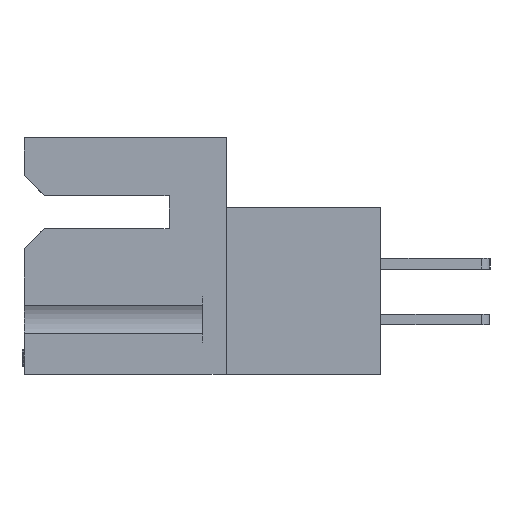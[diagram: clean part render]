
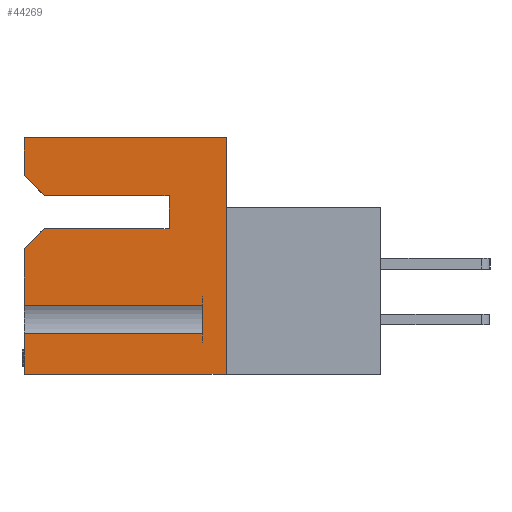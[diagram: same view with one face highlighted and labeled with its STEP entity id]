
A CAD part, left-side view. The second image highlights one B-rep face of the part: STEP entity #44269.
In plain terms, the highlighted planar face has unit normal (-1, 0, 0).
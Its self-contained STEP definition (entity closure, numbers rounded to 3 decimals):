
#11 = CARTESIAN_POINT ( 'NONE',  ( 0., 11.506, -9.556 ) ) ;
#74 = VECTOR ( 'NONE', #31799, 1000. ) ;
#381 = ORIENTED_EDGE ( 'NONE', *, *, #1251, .T. ) ;
#1251 = EDGE_CURVE ( 'NONE', #15625, #25862, #44961, .T. ) ;
#1344 = VECTOR ( 'NONE', #23326, 1000. ) ;
#2158 = VERTEX_POINT ( 'NONE', #34611 ) ;
#2707 = CARTESIAN_POINT ( 'NONE',  ( 0., 0., -5.182 ) ) ;
#2710 = CARTESIAN_POINT ( 'NONE',  ( 0., 11.506, -13.487 ) ) ;
#2832 = DIRECTION ( 'NONE',  ( 0., 1., 0. ) ) ;
#2886 = LINE ( 'NONE', #41673, #43424 ) ;
#2978 = LINE ( 'NONE', #43991, #42972 ) ;
#3442 = ORIENTED_EDGE ( 'NONE', *, *, #13384, .F. ) ;
#3567 = ORIENTED_EDGE ( 'NONE', *, *, #11177, .F. ) ;
#4100 = DIRECTION ( 'NONE',  ( 0., 0., 1. ) ) ;
#4127 = CARTESIAN_POINT ( 'NONE',  ( 0., 11.506, -13.487 ) ) ;
#4578 = VERTEX_POINT ( 'NONE', #9357 ) ;
#4855 = VECTOR ( 'NONE', #24304, 1000. ) ;
#5843 = CARTESIAN_POINT ( 'NONE',  ( 0., 1.346, 0. ) ) ;
#5847 = VERTEX_POINT ( 'NONE', #23316 ) ;
#6884 = CARTESIAN_POINT ( 'NONE',  ( 0., 0., 0. ) ) ;
#7215 = AXIS2_PLACEMENT_3D ( 'NONE', #42971, #36262, #14967 ) ;
#7468 = VERTEX_POINT ( 'NONE', #6884 ) ;
#7484 = EDGE_CURVE ( 'NONE', #35680, #7468, #45311, .T. ) ;
#7867 = EDGE_CURVE ( 'NONE', #18754, #11583, #44698, .T. ) ;
#7870 = VECTOR ( 'NONE', #38408, 1000. ) ;
#8718 = LINE ( 'NONE', #33473, #40984 ) ;
#9357 = CARTESIAN_POINT ( 'NONE',  ( 0., 0., -13.487 ) ) ;
#9514 = LINE ( 'NONE', #14088, #74 ) ;
#10199 = EDGE_CURVE ( 'NONE', #31880, #2158, #37218, .T. ) ;
#10834 = EDGE_CURVE ( 'NONE', #5847, #25862, #2886, .T. ) ;
#11177 = EDGE_CURVE ( 'NONE', #29376, #5847, #9514, .T. ) ;
#11508 = LINE ( 'NONE', #39867, #18219 ) ;
#11583 = VERTEX_POINT ( 'NONE', #40747 ) ;
#11651 = CARTESIAN_POINT ( 'NONE',  ( 0., 11.506, 0. ) ) ;
#13384 = EDGE_CURVE ( 'NONE', #4578, #41341, #16028, .T. ) ;
#14088 = CARTESIAN_POINT ( 'NONE',  ( 0., 3.251, -5.182 ) ) ;
#14967 = DIRECTION ( 'NONE',  ( 0., 0., -1. ) ) ;
#15625 = VERTEX_POINT ( 'NONE', #18851 ) ;
#15901 = DIRECTION ( 'NONE',  ( 0., 0., 1. ) ) ;
#16028 = LINE ( 'NONE', #17100, #24417 ) ;
#17100 = CARTESIAN_POINT ( 'NONE',  ( 0., -8.814, -13.487 ) ) ;
#18219 = VECTOR ( 'NONE', #21829, 1000. ) ;
#18605 = EDGE_CURVE ( 'NONE', #41341, #45968, #33273, .T. ) ;
#18754 = VERTEX_POINT ( 'NONE', #11 ) ;
#18851 = CARTESIAN_POINT ( 'NONE',  ( 0., 11.506, -2.159 ) ) ;
#19410 = EDGE_CURVE ( 'NONE', #7468, #4578, #11508, .T. ) ;
#19704 = ORIENTED_EDGE ( 'NONE', *, *, #19410, .F. ) ;
#20179 = VECTOR ( 'NONE', #40821, 1000. ) ;
#20504 = VECTOR ( 'NONE', #4100, 1000. ) ;
#20573 = DIRECTION ( 'NONE',  ( 0., -1., 0. ) ) ;
#21270 = FACE_OUTER_BOUND ( 'NONE', #30590, .T. ) ;
#21795 = DIRECTION ( 'NONE',  ( 0., 0.707, -0.707 ) ) ;
#21829 = DIRECTION ( 'NONE',  ( 0., 0., -1. ) ) ;
#21961 = PLANE ( 'NONE',  #7215 ) ;
#23316 = CARTESIAN_POINT ( 'NONE',  ( 0., 3.251, -3.302 ) ) ;
#23326 = DIRECTION ( 'NONE',  ( 0., -1., 0. ) ) ;
#23853 = VECTOR ( 'NONE', #27585, 1000. ) ;
#24065 = CARTESIAN_POINT ( 'NONE',  ( 0., 3.251, -5.182 ) ) ;
#24304 = DIRECTION ( 'NONE',  ( 0., -0.707, -0.707 ) ) ;
#24417 = VECTOR ( 'NONE', #2832, 1000. ) ;
#24486 = EDGE_CURVE ( 'NONE', #41481, #11583, #31867, .T. ) ;
#24628 = CARTESIAN_POINT ( 'NONE',  ( 0., 11.506, 0. ) ) ;
#25404 = CARTESIAN_POINT ( 'NONE',  ( 0., 11.506, -13.487 ) ) ;
#25862 = VERTEX_POINT ( 'NONE', #29268 ) ;
#27160 = ORIENTED_EDGE ( 'NONE', *, *, #10199, .T. ) ;
#27585 = DIRECTION ( 'NONE',  ( 0., 0., 1. ) ) ;
#28310 = ORIENTED_EDGE ( 'NONE', *, *, #39598, .F. ) ;
#29268 = CARTESIAN_POINT ( 'NONE',  ( 0., 10.363, -3.302 ) ) ;
#29376 = VERTEX_POINT ( 'NONE', #24065 ) ;
#29701 = VECTOR ( 'NONE', #20573, 1000. ) ;
#29768 = CARTESIAN_POINT ( 'NONE',  ( 0., 1.346, -11.17 ) ) ;
#29977 = LINE ( 'NONE', #25404, #20504 ) ;
#30590 = EDGE_LOOP ( 'NONE', ( #3442, #19704, #40481, #28310, #381, #35959, #3567, #38002, #27160, #40240, #33813, #31810, #33105, #44471 ) ) ;
#31799 = DIRECTION ( 'NONE',  ( 0., 0., 1. ) ) ;
#31810 = ORIENTED_EDGE ( 'NONE', *, *, #24486, .F. ) ;
#31867 = LINE ( 'NONE', #5843, #20179 ) ;
#31880 = VERTEX_POINT ( 'NONE', #42131 ) ;
#33022 = EDGE_CURVE ( 'NONE', #18754, #2158, #8718, .T. ) ;
#33105 = ORIENTED_EDGE ( 'NONE', *, *, #40218, .T. ) ;
#33273 = LINE ( 'NONE', #2710, #23853 ) ;
#33473 = CARTESIAN_POINT ( 'NONE',  ( 0., 11.506, -13.487 ) ) ;
#33813 = ORIENTED_EDGE ( 'NONE', *, *, #7867, .T. ) ;
#34193 = DIRECTION ( 'NONE',  ( 0., 1., 0. ) ) ;
#34611 = CARTESIAN_POINT ( 'NONE',  ( 0., 11.506, -6.325 ) ) ;
#35680 = VERTEX_POINT ( 'NONE', #11651 ) ;
#35959 = ORIENTED_EDGE ( 'NONE', *, *, #10834, .F. ) ;
#36262 = DIRECTION ( 'NONE',  ( 1., 0., 0. ) ) ;
#37218 = LINE ( 'NONE', #39518, #42275 ) ;
#37302 = CARTESIAN_POINT ( 'NONE',  ( 0., 1.346, -9.556 ) ) ;
#38002 = ORIENTED_EDGE ( 'NONE', *, *, #41733, .F. ) ;
#38408 = DIRECTION ( 'NONE',  ( 0., -1., 0. ) ) ;
#39518 = CARTESIAN_POINT ( 'NONE',  ( 0., 10.363, -5.182 ) ) ;
#39598 = EDGE_CURVE ( 'NONE', #15625, #35680, #29977, .T. ) ;
#39867 = CARTESIAN_POINT ( 'NONE',  ( 0., 0., 0. ) ) ;
#40218 = EDGE_CURVE ( 'NONE', #41481, #45968, #2978, .T. ) ;
#40240 = ORIENTED_EDGE ( 'NONE', *, *, #33022, .F. ) ;
#40481 = ORIENTED_EDGE ( 'NONE', *, *, #7484, .F. ) ;
#40747 = CARTESIAN_POINT ( 'NONE',  ( 0., 1.346, -9.556 ) ) ;
#40821 = DIRECTION ( 'NONE',  ( 0., 0., 1. ) ) ;
#40984 = VECTOR ( 'NONE', #15901, 1000. ) ;
#41341 = VERTEX_POINT ( 'NONE', #4127 ) ;
#41481 = VERTEX_POINT ( 'NONE', #29768 ) ;
#41673 = CARTESIAN_POINT ( 'NONE',  ( 0., 0., -3.302 ) ) ;
#41733 = EDGE_CURVE ( 'NONE', #31880, #29376, #42391, .T. ) ;
#41880 = CARTESIAN_POINT ( 'NONE',  ( 0., 10.363, -3.302 ) ) ;
#42131 = CARTESIAN_POINT ( 'NONE',  ( 0., 10.363, -5.182 ) ) ;
#42275 = VECTOR ( 'NONE', #21795, 1000. ) ;
#42391 = LINE ( 'NONE', #2707, #7870 ) ;
#42971 = CARTESIAN_POINT ( 'NONE',  ( 0., 0., 0. ) ) ;
#42972 = VECTOR ( 'NONE', #43837, 1000. ) ;
#43424 = VECTOR ( 'NONE', #34193, 1000. ) ;
#43837 = DIRECTION ( 'NONE',  ( 0., 1., 0. ) ) ;
#43991 = CARTESIAN_POINT ( 'NONE',  ( 0., 1.346, -11.17 ) ) ;
#44269 = ADVANCED_FACE ( 'NONE', ( #21270 ), #21961, .F. ) ;
#44471 = ORIENTED_EDGE ( 'NONE', *, *, #18605, .F. ) ;
#44698 = LINE ( 'NONE', #37302, #1344 ) ;
#44961 = LINE ( 'NONE', #41880, #4855 ) ;
#45311 = LINE ( 'NONE', #24628, #29701 ) ;
#45739 = CARTESIAN_POINT ( 'NONE',  ( 0., 11.506, -11.17 ) ) ;
#45968 = VERTEX_POINT ( 'NONE', #45739 ) ;
